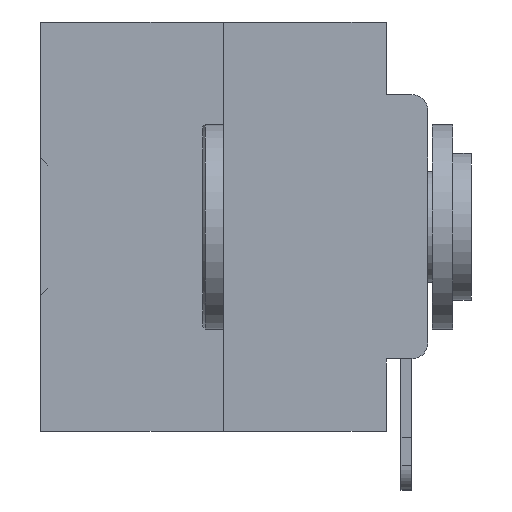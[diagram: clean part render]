
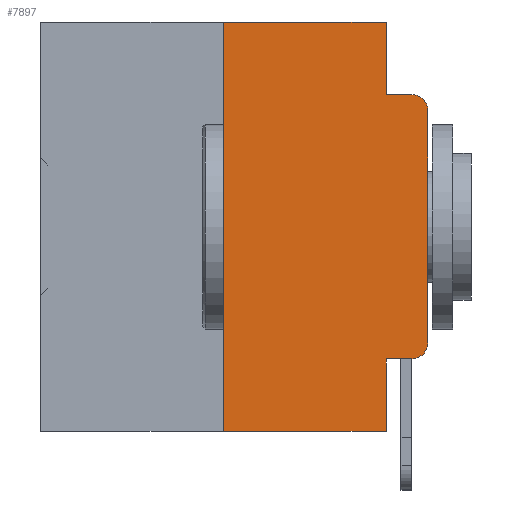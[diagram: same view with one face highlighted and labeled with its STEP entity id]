
A CAD part, left-side view. The second image highlights one B-rep face of the part: STEP entity #7897.
In plain terms, the highlighted planar face has unit normal (-1, 0, 0).
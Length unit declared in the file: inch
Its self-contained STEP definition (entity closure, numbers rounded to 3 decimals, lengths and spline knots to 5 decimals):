
#55 = LINE ( 'NONE', #32507, #20883 ) ;
#88 = ORIENTED_EDGE ( 'NONE', *, *, #34341, .F. ) ;
#265 = DIRECTION ( 'NONE',  ( 0., -1., 0. ) ) ;
#500 = ORIENTED_EDGE ( 'NONE', *, *, #13030, .T. ) ;
#878 = VERTEX_POINT ( 'NONE', #4417 ) ;
#1223 = CARTESIAN_POINT ( 'NONE',  ( 0., 0.473, 0. ) ) ;
#1331 = CARTESIAN_POINT ( 'NONE',  ( 0., 0.051, -0.5 ) ) ;
#1593 = VECTOR ( 'NONE', #9327, 39.37008 ) ;
#2102 = EDGE_CURVE ( 'NONE', #13082, #35725, #6013, .T. ) ;
#2104 = DIRECTION ( 'NONE',  ( 0., 0., 1. ) ) ;
#2225 = CARTESIAN_POINT ( 'NONE',  ( 0., 0.051, -0.4115 ) ) ;
#2324 = AXIS2_PLACEMENT_3D ( 'NONE', #23611, #6007, #26567 ) ;
#2469 = EDGE_LOOP ( 'NONE', ( #500, #10348, #25935, #36237, #88, #10867, #35808, #30946, #32741, #12217 ) ) ;
#2548 = DIRECTION ( 'NONE',  ( 0., 0., -1. ) ) ;
#3323 = LINE ( 'NONE', #26898, #4279 ) ;
#4204 = DIRECTION ( 'NONE',  ( 0., -1., 0. ) ) ;
#4279 = VECTOR ( 'NONE', #9371, 39.37008 ) ;
#4417 = CARTESIAN_POINT ( 'NONE',  ( 0., 0.051, -0.0885 ) ) ;
#4870 = EDGE_CURVE ( 'NONE', #13082, #36163, #27400, .T. ) ;
#4968 = VECTOR ( 'NONE', #2104, 39.37008 ) ;
#5376 = LINE ( 'NONE', #17087, #35476 ) ;
#5989 = CARTESIAN_POINT ( 'NONE',  ( 0., 0.25, 0. ) ) ;
#6007 = DIRECTION ( 'NONE',  ( 1., 0., 0. ) ) ;
#6013 = LINE ( 'NONE', #10097, #28526 ) ;
#6252 = FACE_OUTER_BOUND ( 'NONE', #2469, .T. ) ;
#6674 = EDGE_CURVE ( 'NONE', #30560, #33468, #3323, .T. ) ;
#7897 = ADVANCED_FACE ( 'NONE', ( #6252 ), #18595, .F. ) ;
#9125 = EDGE_CURVE ( 'NONE', #30560, #35725, #34028, .T. ) ;
#9152 = VERTEX_POINT ( 'NONE', #28767 ) ;
#9327 = DIRECTION ( 'NONE',  ( 0., -1., 0. ) ) ;
#9371 = DIRECTION ( 'NONE',  ( 0., 0., 1. ) ) ;
#9900 = VECTOR ( 'NONE', #17027, 39.37008 ) ;
#10097 = CARTESIAN_POINT ( 'NONE',  ( 0., 0.051, 0. ) ) ;
#10117 = CIRCLE ( 'NONE', #14427, 0.02 ) ;
#10348 = ORIENTED_EDGE ( 'NONE', *, *, #37090, .T. ) ;
#10822 = LINE ( 'NONE', #1223, #18576 ) ;
#10867 = ORIENTED_EDGE ( 'NONE', *, *, #6674, .F. ) ;
#12135 = CARTESIAN_POINT ( 'NONE',  ( 0., 0.051, -0.4115 ) ) ;
#12217 = ORIENTED_EDGE ( 'NONE', *, *, #36596, .T. ) ;
#13030 = EDGE_CURVE ( 'NONE', #33573, #15669, #25653, .T. ) ;
#13082 = VERTEX_POINT ( 'NONE', #2225 ) ;
#14080 = CARTESIAN_POINT ( 'NONE',  ( 0., 0.473, -0.5 ) ) ;
#14427 = AXIS2_PLACEMENT_3D ( 'NONE', #34151, #16791, #36968 ) ;
#14823 = CARTESIAN_POINT ( 'NONE',  ( 0., 0., -0.1085 ) ) ;
#15669 = VERTEX_POINT ( 'NONE', #14823 ) ;
#16791 = DIRECTION ( 'NONE',  ( -1., 0., 0. ) ) ;
#16833 = CARTESIAN_POINT ( 'NONE',  ( 0., 0.051, 0. ) ) ;
#17027 = DIRECTION ( 'NONE',  ( 0., -1., 0. ) ) ;
#17087 = CARTESIAN_POINT ( 'NONE',  ( 0., 0.051, 0. ) ) ;
#18340 = CARTESIAN_POINT ( 'NONE',  ( 0., 0., -0.3915 ) ) ;
#18576 = VECTOR ( 'NONE', #4204, 39.37008 ) ;
#18595 = PLANE ( 'NONE',  #2324 ) ;
#19779 = CIRCLE ( 'NONE', #23696, 0.02 ) ;
#20271 = DIRECTION ( 'NONE',  ( -1., 0., 0. ) ) ;
#20717 = EDGE_CURVE ( 'NONE', #878, #9152, #55, .T. ) ;
#20883 = VECTOR ( 'NONE', #265, 39.37008 ) ;
#22246 = CARTESIAN_POINT ( 'NONE',  ( 0., 0.25, -0.5 ) ) ;
#22746 = CARTESIAN_POINT ( 'NONE',  ( 0., 0., 0. ) ) ;
#23611 = CARTESIAN_POINT ( 'NONE',  ( 0., 0.473, 0. ) ) ;
#23696 = AXIS2_PLACEMENT_3D ( 'NONE', #37523, #20271, #2548 ) ;
#23980 = CARTESIAN_POINT ( 'NONE',  ( 0., 0.02, -0.4115 ) ) ;
#24525 = DIRECTION ( 'NONE',  ( 0., 0., -1. ) ) ;
#25653 = LINE ( 'NONE', #22746, #4968 ) ;
#25935 = ORIENTED_EDGE ( 'NONE', *, *, #20717, .F. ) ;
#26320 = EDGE_CURVE ( 'NONE', #36505, #878, #5376, .T. ) ;
#26567 = DIRECTION ( 'NONE',  ( 0., 0., -1. ) ) ;
#26898 = CARTESIAN_POINT ( 'NONE',  ( 0., 0.25, 0. ) ) ;
#27400 = LINE ( 'NONE', #12135, #1593 ) ;
#28526 = VECTOR ( 'NONE', #24525, 39.37008 ) ;
#28767 = CARTESIAN_POINT ( 'NONE',  ( 0., 0.02, -0.0885 ) ) ;
#30560 = VERTEX_POINT ( 'NONE', #22246 ) ;
#30946 = ORIENTED_EDGE ( 'NONE', *, *, #2102, .F. ) ;
#31606 = DIRECTION ( 'NONE',  ( 0., 0., -1. ) ) ;
#32507 = CARTESIAN_POINT ( 'NONE',  ( 0., 0.051, -0.0885 ) ) ;
#32741 = ORIENTED_EDGE ( 'NONE', *, *, #4870, .T. ) ;
#33468 = VERTEX_POINT ( 'NONE', #5989 ) ;
#33573 = VERTEX_POINT ( 'NONE', #18340 ) ;
#34028 = LINE ( 'NONE', #14080, #9900 ) ;
#34151 = CARTESIAN_POINT ( 'NONE',  ( 0., 0.02, -0.1085 ) ) ;
#34341 = EDGE_CURVE ( 'NONE', #33468, #36505, #10822, .T. ) ;
#35476 = VECTOR ( 'NONE', #31606, 39.37008 ) ;
#35725 = VERTEX_POINT ( 'NONE', #1331 ) ;
#35808 = ORIENTED_EDGE ( 'NONE', *, *, #9125, .T. ) ;
#36163 = VERTEX_POINT ( 'NONE', #23980 ) ;
#36237 = ORIENTED_EDGE ( 'NONE', *, *, #26320, .F. ) ;
#36505 = VERTEX_POINT ( 'NONE', #16833 ) ;
#36596 = EDGE_CURVE ( 'NONE', #36163, #33573, #19779, .T. ) ;
#36968 = DIRECTION ( 'NONE',  ( 0., 0., -1. ) ) ;
#37090 = EDGE_CURVE ( 'NONE', #15669, #9152, #10117, .T. ) ;
#37523 = CARTESIAN_POINT ( 'NONE',  ( 0., 0.02, -0.3915 ) ) ;
